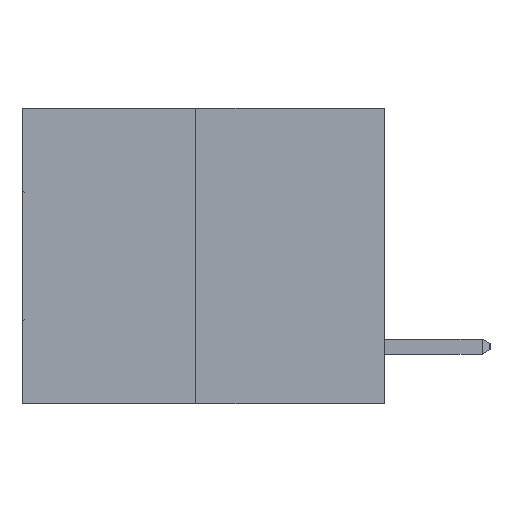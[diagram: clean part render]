
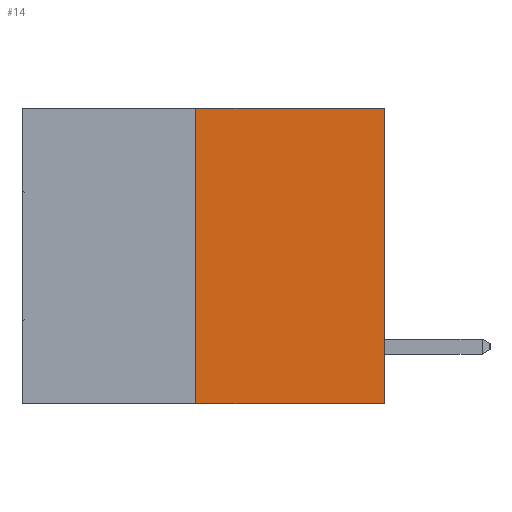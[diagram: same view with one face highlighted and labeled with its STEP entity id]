
A CAD part, left-side view. The second image highlights one B-rep face of the part: STEP entity #14.
In plain terms, the highlighted planar face has unit normal (-1, 0, 0).
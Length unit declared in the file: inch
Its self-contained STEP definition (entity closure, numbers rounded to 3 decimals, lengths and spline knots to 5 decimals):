
#14 = ADVANCED_FACE ( 'NONE', ( #26083 ), #26931, .F. ) ;
#1216 = EDGE_CURVE ( 'NONE', #20827, #19313, #2855, .T. ) ;
#1841 = ORIENTED_EDGE ( 'NONE', *, *, #1216, .F. ) ;
#2855 = LINE ( 'NONE', #5253, #22384 ) ;
#4476 = CARTESIAN_POINT ( 'NONE',  ( 0., 0.312, -0.49 ) ) ;
#5185 = EDGE_LOOP ( 'NONE', ( #1841, #9848, #17462, #22607 ) ) ;
#5253 = CARTESIAN_POINT ( 'NONE',  ( 0., 0.312, -0.49 ) ) ;
#5684 = VERTEX_POINT ( 'NONE', #13314 ) ;
#7176 = CARTESIAN_POINT ( 'NONE',  ( 0., 0., 0. ) ) ;
#8651 = DIRECTION ( 'NONE',  ( 0., 0., 1. ) ) ;
#9055 = VECTOR ( 'NONE', #8651, 39.37008 ) ;
#9848 = ORIENTED_EDGE ( 'NONE', *, *, #23214, .T. ) ;
#10955 = CARTESIAN_POINT ( 'NONE',  ( 0., 0., 0. ) ) ;
#11715 = VECTOR ( 'NONE', #32279, 39.37008 ) ;
#13314 = CARTESIAN_POINT ( 'NONE',  ( 0., 0., -0.49 ) ) ;
#13328 = DIRECTION ( 'NONE',  ( 0., -1., 0. ) ) ;
#15596 = CARTESIAN_POINT ( 'NONE',  ( 0., 0.6, -0.49 ) ) ;
#16207 = VECTOR ( 'NONE', #13328, 39.37008 ) ;
#17462 = ORIENTED_EDGE ( 'NONE', *, *, #32075, .T. ) ;
#17757 = CARTESIAN_POINT ( 'NONE',  ( 0., 0.312, 0. ) ) ;
#18499 = EDGE_CURVE ( 'NONE', #19313, #30600, #18558, .T. ) ;
#18558 = LINE ( 'NONE', #29948, #11715 ) ;
#19313 = VERTEX_POINT ( 'NONE', #17757 ) ;
#19320 = CARTESIAN_POINT ( 'NONE',  ( 0., 0.6, 0. ) ) ;
#19437 = DIRECTION ( 'NONE',  ( 1., 0., 0. ) ) ;
#20233 = LINE ( 'NONE', #10955, #9055 ) ;
#20630 = DIRECTION ( 'NONE',  ( 0., 0., 1. ) ) ;
#20827 = VERTEX_POINT ( 'NONE', #4476 ) ;
#21028 = AXIS2_PLACEMENT_3D ( 'NONE', #19320, #19437, #29739 ) ;
#22384 = VECTOR ( 'NONE', #20630, 39.37008 ) ;
#22562 = LINE ( 'NONE', #15596, #16207 ) ;
#22607 = ORIENTED_EDGE ( 'NONE', *, *, #18499, .F. ) ;
#23214 = EDGE_CURVE ( 'NONE', #20827, #5684, #22562, .T. ) ;
#26083 = FACE_OUTER_BOUND ( 'NONE', #5185, .T. ) ;
#26931 = PLANE ( 'NONE',  #21028 ) ;
#29739 = DIRECTION ( 'NONE',  ( 0., 0., -1. ) ) ;
#29948 = CARTESIAN_POINT ( 'NONE',  ( 0., 0.6, 0. ) ) ;
#30600 = VERTEX_POINT ( 'NONE', #7176 ) ;
#32075 = EDGE_CURVE ( 'NONE', #5684, #30600, #20233, .T. ) ;
#32279 = DIRECTION ( 'NONE',  ( 0., -1., 0. ) ) ;
